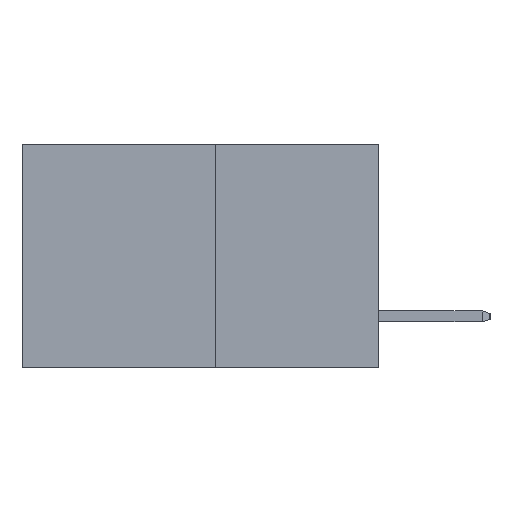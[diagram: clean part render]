
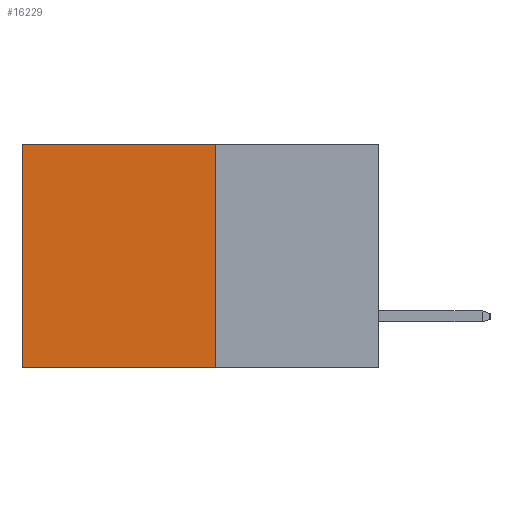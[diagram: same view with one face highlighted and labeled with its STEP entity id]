
A CAD part, left-side view. The second image highlights one B-rep face of the part: STEP entity #16229.
In plain terms, the highlighted planar face has unit normal (-1, 0, 0).
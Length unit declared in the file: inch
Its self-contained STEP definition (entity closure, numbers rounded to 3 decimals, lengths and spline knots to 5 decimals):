
#266 = CARTESIAN_POINT ( 'NONE',  ( 0.277, 0.59, -0.37 ) ) ;
#368 = CARTESIAN_POINT ( 'NONE',  ( 0.277, 0.27, 0. ) ) ;
#888 = LINE ( 'NONE', #368, #19271 ) ;
#1545 = DIRECTION ( 'NONE',  ( 0., 0., -1. ) ) ;
#2270 = DIRECTION ( 'NONE',  ( 0., 0., -1. ) ) ;
#2318 = CARTESIAN_POINT ( 'NONE',  ( 0.277, 0.59, 0. ) ) ;
#3467 = DIRECTION ( 'NONE',  ( 0., 0., -1. ) ) ;
#3696 = VECTOR ( 'NONE', #2270, 39.37008 ) ;
#4439 = LINE ( 'NONE', #14420, #9313 ) ;
#5846 = ORIENTED_EDGE ( 'NONE', *, *, #8751, .F. ) ;
#6017 = AXIS2_PLACEMENT_3D ( 'NONE', #10661, #12523, #1545 ) ;
#6539 = CARTESIAN_POINT ( 'NONE',  ( 0.277, 0.27, 0. ) ) ;
#6900 = CARTESIAN_POINT ( 'NONE',  ( 0.277, 0.27, -0.37 ) ) ;
#6944 = CARTESIAN_POINT ( 'NONE',  ( 0.277, 0.27, -0.37 ) ) ;
#7073 = ORIENTED_EDGE ( 'NONE', *, *, #13286, .T. ) ;
#7461 = EDGE_CURVE ( 'NONE', #16746, #17476, #4439, .T. ) ;
#8751 = EDGE_CURVE ( 'NONE', #17476, #15921, #9614, .T. ) ;
#9313 = VECTOR ( 'NONE', #3467, 39.37008 ) ;
#9419 = VERTEX_POINT ( 'NONE', #2318 ) ;
#9614 = LINE ( 'NONE', #6944, #22948 ) ;
#9730 = ORIENTED_EDGE ( 'NONE', *, *, #17142, .T. ) ;
#10661 = CARTESIAN_POINT ( 'NONE',  ( 0.277, 0.27, -0.37 ) ) ;
#12523 = DIRECTION ( 'NONE',  ( 1., 0., 0. ) ) ;
#13286 = EDGE_CURVE ( 'NONE', #9419, #15921, #13425, .T. ) ;
#13376 = DIRECTION ( 'NONE',  ( 0., 1., 0. ) ) ;
#13425 = LINE ( 'NONE', #266, #3696 ) ;
#13501 = EDGE_LOOP ( 'NONE', ( #7073, #5846, #18786, #9730 ) ) ;
#14420 = CARTESIAN_POINT ( 'NONE',  ( 0.277, 0.27, -0.37 ) ) ;
#14463 = FACE_OUTER_BOUND ( 'NONE', #13501, .T. ) ;
#15921 = VERTEX_POINT ( 'NONE', #20802 ) ;
#16229 = ADVANCED_FACE ( 'NONE', ( #14463 ), #21569, .F. ) ;
#16746 = VERTEX_POINT ( 'NONE', #6539 ) ;
#17142 = EDGE_CURVE ( 'NONE', #16746, #9419, #888, .T. ) ;
#17476 = VERTEX_POINT ( 'NONE', #6900 ) ;
#17872 = DIRECTION ( 'NONE',  ( 0., 1., 0. ) ) ;
#18786 = ORIENTED_EDGE ( 'NONE', *, *, #7461, .F. ) ;
#19271 = VECTOR ( 'NONE', #13376, 39.37008 ) ;
#20802 = CARTESIAN_POINT ( 'NONE',  ( 0.277, 0.59, -0.37 ) ) ;
#21569 = PLANE ( 'NONE',  #6017 ) ;
#22948 = VECTOR ( 'NONE', #17872, 39.37008 ) ;
